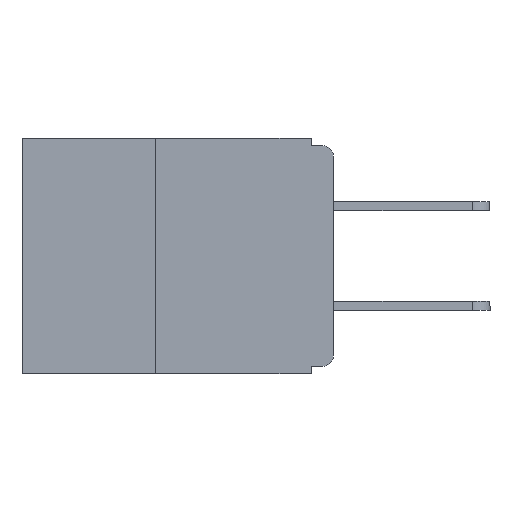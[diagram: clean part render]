
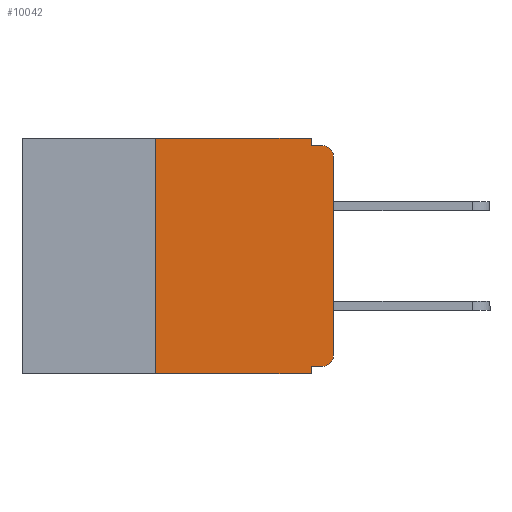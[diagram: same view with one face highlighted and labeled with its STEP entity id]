
A CAD part, left-side view. The second image highlights one B-rep face of the part: STEP entity #10042.
In plain terms, the highlighted planar face has unit normal (-1, 0, 0).
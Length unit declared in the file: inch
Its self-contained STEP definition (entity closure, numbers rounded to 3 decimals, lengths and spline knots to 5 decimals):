
#145 = DIRECTION ( 'NONE',  ( 0., -1., 0. ) ) ;
#188 = CARTESIAN_POINT ( 'NONE',  ( 0., 0.25, -0.33 ) ) ;
#200 = ORIENTED_EDGE ( 'NONE', *, *, #14435, .F. ) ;
#384 = ORIENTED_EDGE ( 'NONE', *, *, #23554, .F. ) ;
#387 = DIRECTION ( 'NONE',  ( 0., 0., -1. ) ) ;
#538 = VECTOR ( 'NONE', #859, 39.37008 ) ;
#859 = DIRECTION ( 'NONE',  ( 0., 0., -1. ) ) ;
#1648 = LINE ( 'NONE', #14432, #11634 ) ;
#1656 = VECTOR ( 'NONE', #145, 39.37008 ) ;
#1832 = ORIENTED_EDGE ( 'NONE', *, *, #15903, .F. ) ;
#1955 = ORIENTED_EDGE ( 'NONE', *, *, #22360, .F. ) ;
#1957 = EDGE_CURVE ( 'NONE', #23507, #2092, #11240, .T. ) ;
#1969 = CARTESIAN_POINT ( 'NONE',  ( 0., 0.031, 0. ) ) ;
#2004 = VECTOR ( 'NONE', #22855, 39.37008 ) ;
#2092 = VERTEX_POINT ( 'NONE', #5247 ) ;
#2195 = ORIENTED_EDGE ( 'NONE', *, *, #19944, .T. ) ;
#2786 = ORIENTED_EDGE ( 'NONE', *, *, #5722, .T. ) ;
#3021 = ORIENTED_EDGE ( 'NONE', *, *, #18740, .F. ) ;
#3280 = DIRECTION ( 'NONE',  ( 0., -1., 0. ) ) ;
#3830 = ORIENTED_EDGE ( 'NONE', *, *, #9516, .F. ) ;
#3888 = LINE ( 'NONE', #11636, #12698 ) ;
#3926 = ORIENTED_EDGE ( 'NONE', *, *, #1957, .T. ) ;
#5089 = LINE ( 'NONE', #8039, #14393 ) ;
#5244 = EDGE_CURVE ( 'NONE', #2092, #23241, #16227, .T. ) ;
#5247 = CARTESIAN_POINT ( 'NONE',  ( 0., 0., -0.305 ) ) ;
#5722 = EDGE_CURVE ( 'NONE', #23241, #15222, #20524, .T. ) ;
#5808 = CARTESIAN_POINT ( 'NONE',  ( 0., 0.015, -0.32 ) ) ;
#6250 = CARTESIAN_POINT ( 'NONE',  ( 0., 0.031, -0.33 ) ) ;
#6502 = VERTEX_POINT ( 'NONE', #8058 ) ;
#6633 = LINE ( 'NONE', #14974, #1656 ) ;
#7182 = ORIENTED_EDGE ( 'NONE', *, *, #5244, .T. ) ;
#7506 = AXIS2_PLACEMENT_3D ( 'NONE', #9992, #22766, #11865 ) ;
#7643 = DIRECTION ( 'NONE',  ( 0., 0., -1. ) ) ;
#8039 = CARTESIAN_POINT ( 'NONE',  ( 0., 0., -0.32 ) ) ;
#8058 = CARTESIAN_POINT ( 'NONE',  ( 0., 0.25, -0.33 ) ) ;
#8314 = FACE_OUTER_BOUND ( 'NONE', #20220, .T. ) ;
#8329 = CARTESIAN_POINT ( 'NONE',  ( 0., 0.031, -0.33 ) ) ;
#9282 = VERTEX_POINT ( 'NONE', #20181 ) ;
#9426 = CARTESIAN_POINT ( 'NONE',  ( 0., 0.015, -0.01 ) ) ;
#9516 = EDGE_CURVE ( 'NONE', #23507, #9282, #5089, .T. ) ;
#9933 = DIRECTION ( 'NONE',  ( 0., 1., 0. ) ) ;
#9992 = CARTESIAN_POINT ( 'NONE',  ( 0., 0.437, 0. ) ) ;
#10042 = ADVANCED_FACE ( 'NONE', ( #8314 ), #15425, .F. ) ;
#10534 = LINE ( 'NONE', #8329, #538 ) ;
#10756 = VERTEX_POINT ( 'NONE', #11736 ) ;
#11240 = CIRCLE ( 'NONE', #17565, 0.015 ) ;
#11634 = VECTOR ( 'NONE', #3280, 39.37008 ) ;
#11636 = CARTESIAN_POINT ( 'NONE',  ( 0., 0.031, 0. ) ) ;
#11736 = CARTESIAN_POINT ( 'NONE',  ( 0., 0.25, 0. ) ) ;
#11865 = DIRECTION ( 'NONE',  ( 0., 0., -1. ) ) ;
#12698 = VECTOR ( 'NONE', #387, 39.37008 ) ;
#14108 = AXIS2_PLACEMENT_3D ( 'NONE', #15776, #15722, #15941 ) ;
#14358 = LINE ( 'NONE', #16847, #19260 ) ;
#14393 = VECTOR ( 'NONE', #9933, 39.37008 ) ;
#14432 = CARTESIAN_POINT ( 'NONE',  ( 0., 0., -0.01 ) ) ;
#14435 = EDGE_CURVE ( 'NONE', #16420, #15222, #1648, .T. ) ;
#14708 = LINE ( 'NONE', #188, #23797 ) ;
#14974 = CARTESIAN_POINT ( 'NONE',  ( 0., 0.437, -0.33 ) ) ;
#15094 = CARTESIAN_POINT ( 'NONE',  ( 0., 0.015, -0.305 ) ) ;
#15095 = DIRECTION ( 'NONE',  ( 0., 0., 1. ) ) ;
#15222 = VERTEX_POINT ( 'NONE', #9426 ) ;
#15425 = PLANE ( 'NONE',  #7506 ) ;
#15722 = DIRECTION ( 'NONE',  ( -1., 0., 0. ) ) ;
#15776 = CARTESIAN_POINT ( 'NONE',  ( 0., 0.015, -0.025 ) ) ;
#15903 = EDGE_CURVE ( 'NONE', #10756, #17867, #14358, .T. ) ;
#15941 = DIRECTION ( 'NONE',  ( 0., 0., -1. ) ) ;
#16227 = LINE ( 'NONE', #22089, #2004 ) ;
#16420 = VERTEX_POINT ( 'NONE', #17755 ) ;
#16847 = CARTESIAN_POINT ( 'NONE',  ( 0., 0.437, 0. ) ) ;
#17565 = AXIS2_PLACEMENT_3D ( 'NONE', #15094, #18365, #7643 ) ;
#17755 = CARTESIAN_POINT ( 'NONE',  ( 0., 0.031, -0.01 ) ) ;
#17867 = VERTEX_POINT ( 'NONE', #1969 ) ;
#18365 = DIRECTION ( 'NONE',  ( -1., 0., 0. ) ) ;
#18716 = DIRECTION ( 'NONE',  ( 0., -1., 0. ) ) ;
#18740 = EDGE_CURVE ( 'NONE', #9282, #19489, #10534, .T. ) ;
#19260 = VECTOR ( 'NONE', #18716, 39.37008 ) ;
#19489 = VERTEX_POINT ( 'NONE', #6250 ) ;
#19944 = EDGE_CURVE ( 'NONE', #6502, #19489, #6633, .T. ) ;
#20181 = CARTESIAN_POINT ( 'NONE',  ( 0., 0.031, -0.32 ) ) ;
#20220 = EDGE_LOOP ( 'NONE', ( #7182, #2786, #200, #384, #1832, #1955, #2195, #3021, #3830, #3926 ) ) ;
#20524 = CIRCLE ( 'NONE', #14108, 0.015 ) ;
#21522 = CARTESIAN_POINT ( 'NONE',  ( 0., 0., -0.025 ) ) ;
#22089 = CARTESIAN_POINT ( 'NONE',  ( 0., 0., 0. ) ) ;
#22360 = EDGE_CURVE ( 'NONE', #6502, #10756, #14708, .T. ) ;
#22766 = DIRECTION ( 'NONE',  ( 1., 0., 0. ) ) ;
#22855 = DIRECTION ( 'NONE',  ( 0., 0., 1. ) ) ;
#23241 = VERTEX_POINT ( 'NONE', #21522 ) ;
#23507 = VERTEX_POINT ( 'NONE', #5808 ) ;
#23554 = EDGE_CURVE ( 'NONE', #17867, #16420, #3888, .T. ) ;
#23797 = VECTOR ( 'NONE', #15095, 39.37008 ) ;
